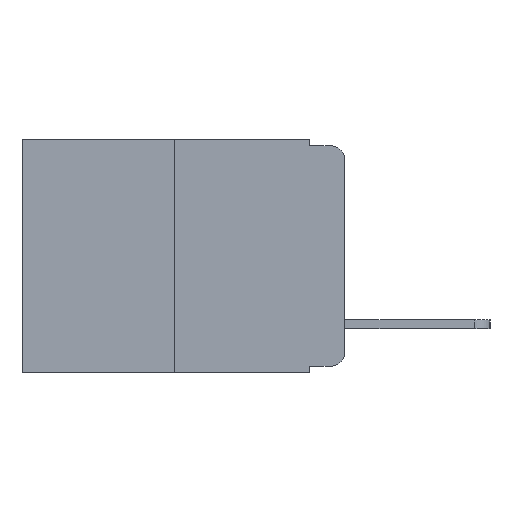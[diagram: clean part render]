
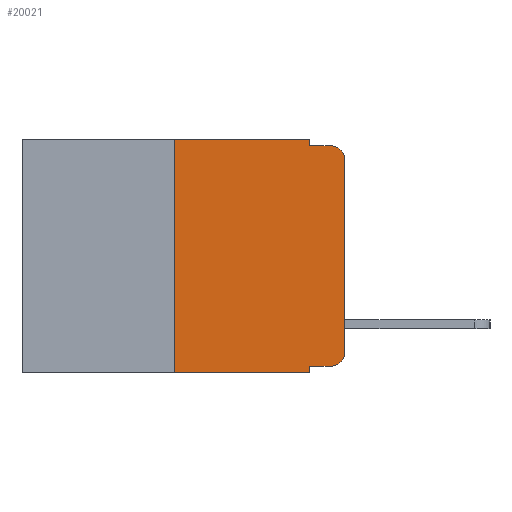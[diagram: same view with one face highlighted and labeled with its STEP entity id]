
A CAD part, left-side view. The second image highlights one B-rep face of the part: STEP entity #20021.
In plain terms, the highlighted planar face has unit normal (-1, 0, 0).
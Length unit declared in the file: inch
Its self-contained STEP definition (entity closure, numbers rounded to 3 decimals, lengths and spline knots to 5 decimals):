
#77 = EDGE_CURVE ( 'NONE', #19460, #19193, #8675, .T. ) ;
#91 = CARTESIAN_POINT ( 'NONE',  ( 0., 0.051, -0.01 ) ) ;
#115 = EDGE_CURVE ( 'NONE', #1617, #16982, #11348, .T. ) ;
#180 = ORIENTED_EDGE ( 'NONE', *, *, #13357, .T. ) ;
#680 = VERTEX_POINT ( 'NONE', #18564 ) ;
#743 = ORIENTED_EDGE ( 'NONE', *, *, #115, .F. ) ;
#957 = DIRECTION ( 'NONE',  ( 0., 0., -1. ) ) ;
#1275 = EDGE_CURVE ( 'NONE', #19460, #4073, #2561, .T. ) ;
#1357 = DIRECTION ( 'NONE',  ( 1., 0., 0. ) ) ;
#1443 = ORIENTED_EDGE ( 'NONE', *, *, #17441, .F. ) ;
#1617 = VERTEX_POINT ( 'NONE', #19650 ) ;
#1676 = AXIS2_PLACEMENT_3D ( 'NONE', #9390, #1357, #12492 ) ;
#1819 = ORIENTED_EDGE ( 'NONE', *, *, #1275, .F. ) ;
#2154 = CARTESIAN_POINT ( 'NONE',  ( 0., 0.051, 0. ) ) ;
#2492 = CARTESIAN_POINT ( 'NONE',  ( 0., 0.051, 0. ) ) ;
#2561 = LINE ( 'NONE', #2492, #6368 ) ;
#3578 = AXIS2_PLACEMENT_3D ( 'NONE', #18898, #9756, #10475 ) ;
#4073 = VERTEX_POINT ( 'NONE', #15828 ) ;
#4594 = ORIENTED_EDGE ( 'NONE', *, *, #14331, .F. ) ;
#4897 = VECTOR ( 'NONE', #7723, 39.37008 ) ;
#5684 = CARTESIAN_POINT ( 'NONE',  ( 0., 0.051, -0.01 ) ) ;
#6006 = VERTEX_POINT ( 'NONE', #16728 ) ;
#6368 = VECTOR ( 'NONE', #957, 39.37008 ) ;
#6444 = VECTOR ( 'NONE', #9116, 39.37008 ) ;
#6579 = CARTESIAN_POINT ( 'NONE',  ( 0., 0.051, 0. ) ) ;
#6653 = VECTOR ( 'NONE', #18317, 39.37008 ) ;
#7176 = VECTOR ( 'NONE', #16926, 39.37008 ) ;
#7231 = CARTESIAN_POINT ( 'NONE',  ( 0., 0.051, -0.333 ) ) ;
#7255 = LINE ( 'NONE', #91, #11901 ) ;
#7272 = DIRECTION ( 'NONE',  ( -1., 0., 0. ) ) ;
#7723 = DIRECTION ( 'NONE',  ( 0., -1., 0. ) ) ;
#7783 = CARTESIAN_POINT ( 'NONE',  ( 0., 0., 0. ) ) ;
#7808 = PLANE ( 'NONE',  #1676 ) ;
#8675 = LINE ( 'NONE', #7231, #4897 ) ;
#9116 = DIRECTION ( 'NONE',  ( 0., -1., 0. ) ) ;
#9390 = CARTESIAN_POINT ( 'NONE',  ( 0., 0.473, 0. ) ) ;
#9528 = AXIS2_PLACEMENT_3D ( 'NONE', #16477, #7272, #18033 ) ;
#9756 = DIRECTION ( 'NONE',  ( -1., 0., 0. ) ) ;
#9803 = CIRCLE ( 'NONE', #3578, 0.02 ) ;
#9844 = DIRECTION ( 'NONE',  ( 0., -1., 0. ) ) ;
#9932 = CARTESIAN_POINT ( 'NONE',  ( 0., 0., -0.03 ) ) ;
#10359 = ORIENTED_EDGE ( 'NONE', *, *, #15556, .T. ) ;
#10475 = DIRECTION ( 'NONE',  ( 0., 0., -1. ) ) ;
#10958 = DIRECTION ( 'NONE',  ( 0., 0., 1. ) ) ;
#11259 = CARTESIAN_POINT ( 'NONE',  ( 0., 0.051, -0.333 ) ) ;
#11325 = LINE ( 'NONE', #15208, #6653 ) ;
#11348 = LINE ( 'NONE', #16983, #7176 ) ;
#11804 = ORIENTED_EDGE ( 'NONE', *, *, #15379, .F. ) ;
#11901 = VECTOR ( 'NONE', #9844, 39.37008 ) ;
#12344 = EDGE_CURVE ( 'NONE', #6006, #20241, #13359, .T. ) ;
#12492 = DIRECTION ( 'NONE',  ( 0., 0., -1. ) ) ;
#12916 = FACE_OUTER_BOUND ( 'NONE', #17714, .T. ) ;
#13357 = EDGE_CURVE ( 'NONE', #20241, #680, #18099, .T. ) ;
#13359 = LINE ( 'NONE', #7783, #16931 ) ;
#13921 = VERTEX_POINT ( 'NONE', #5684 ) ;
#13945 = LINE ( 'NONE', #2154, #17566 ) ;
#14331 = EDGE_CURVE ( 'NONE', #13921, #680, #7255, .T. ) ;
#14835 = ORIENTED_EDGE ( 'NONE', *, *, #77, .T. ) ;
#15208 = CARTESIAN_POINT ( 'NONE',  ( 0., 0.25, 0. ) ) ;
#15379 = EDGE_CURVE ( 'NONE', #16982, #13921, #13945, .T. ) ;
#15556 = EDGE_CURVE ( 'NONE', #16120, #4073, #19220, .T. ) ;
#15828 = CARTESIAN_POINT ( 'NONE',  ( 0., 0.051, -0.343 ) ) ;
#16120 = VERTEX_POINT ( 'NONE', #18403 ) ;
#16477 = CARTESIAN_POINT ( 'NONE',  ( 0., 0.02, -0.03 ) ) ;
#16728 = CARTESIAN_POINT ( 'NONE',  ( 0., 0., -0.313 ) ) ;
#16926 = DIRECTION ( 'NONE',  ( 0., -1., 0. ) ) ;
#16931 = VECTOR ( 'NONE', #10958, 39.37008 ) ;
#16982 = VERTEX_POINT ( 'NONE', #6579 ) ;
#16983 = CARTESIAN_POINT ( 'NONE',  ( 0., 0.473, 0. ) ) ;
#17441 = EDGE_CURVE ( 'NONE', #16120, #1617, #11325, .T. ) ;
#17566 = VECTOR ( 'NONE', #19283, 39.37008 ) ;
#17569 = ORIENTED_EDGE ( 'NONE', *, *, #19490, .T. ) ;
#17714 = EDGE_LOOP ( 'NONE', ( #19876, #180, #4594, #11804, #743, #1443, #10359, #1819, #14835, #17569 ) ) ;
#18033 = DIRECTION ( 'NONE',  ( 0., 0., -1. ) ) ;
#18099 = CIRCLE ( 'NONE', #9528, 0.02 ) ;
#18188 = CARTESIAN_POINT ( 'NONE',  ( 0., 0.02, -0.333 ) ) ;
#18291 = CARTESIAN_POINT ( 'NONE',  ( 0., 0.473, -0.343 ) ) ;
#18317 = DIRECTION ( 'NONE',  ( 0., 0., 1. ) ) ;
#18403 = CARTESIAN_POINT ( 'NONE',  ( 0., 0.25, -0.343 ) ) ;
#18564 = CARTESIAN_POINT ( 'NONE',  ( 0., 0.02, -0.01 ) ) ;
#18898 = CARTESIAN_POINT ( 'NONE',  ( 0., 0.02, -0.313 ) ) ;
#19193 = VERTEX_POINT ( 'NONE', #18188 ) ;
#19220 = LINE ( 'NONE', #18291, #6444 ) ;
#19283 = DIRECTION ( 'NONE',  ( 0., 0., -1. ) ) ;
#19460 = VERTEX_POINT ( 'NONE', #11259 ) ;
#19490 = EDGE_CURVE ( 'NONE', #19193, #6006, #9803, .T. ) ;
#19650 = CARTESIAN_POINT ( 'NONE',  ( 0., 0.25, 0. ) ) ;
#19876 = ORIENTED_EDGE ( 'NONE', *, *, #12344, .T. ) ;
#20021 = ADVANCED_FACE ( 'NONE', ( #12916 ), #7808, .F. ) ;
#20241 = VERTEX_POINT ( 'NONE', #9932 ) ;
